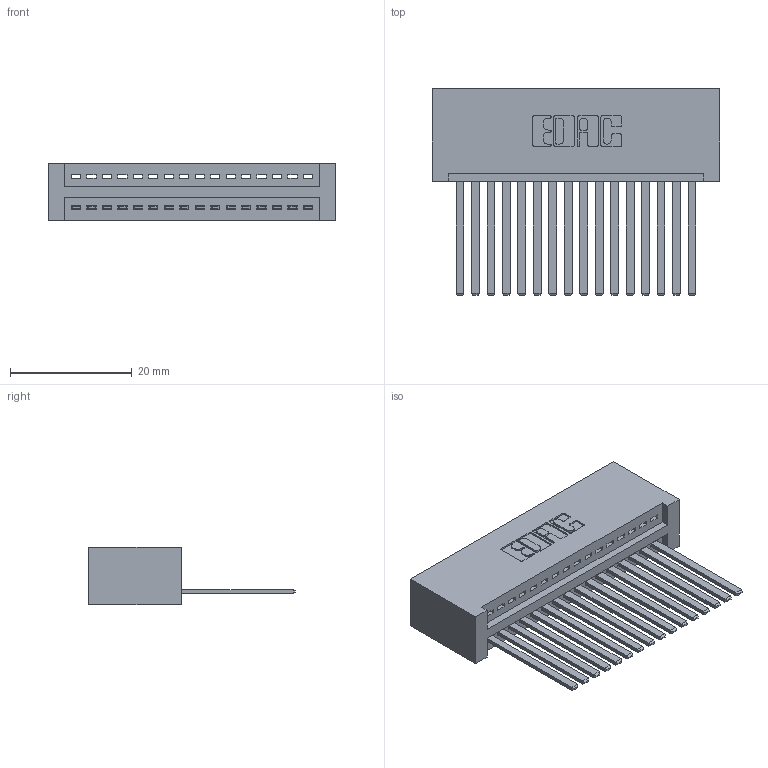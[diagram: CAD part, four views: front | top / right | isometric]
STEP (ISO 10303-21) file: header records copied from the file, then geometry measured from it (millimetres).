
FILE_DESCRIPTION (( 'STEP AP203' ), '1' );
FILE_NAME ('345-016-544-101.STEP', '2018-08-19T00:21:24', ( '' ), ( '' ), 'SwSTEP 2.0', 'SolidWorks 2016', '' );
FILE_SCHEMA (( 'CONFIG_CONTROL_DESIGN' ));
Length unit declared in the file: inch
Products named in the file (3): 345 Part_No Mounting Lugs; 345-292-001_345-293-144; 345-016-544-101
Assembly tree (17 placements, depth 2):
  345-016-544-101
    345 Part_No Mounting Lugs
    345-292-001_345-293-144  x16
Bounding box: 47.24 x 33.96 x 9.4 mm (x, y, z)
Volume: 5044 mm3; surface area: 7096 mm2
Topology: 17 solids, 17 shells, 950 faces, 2845 edges, 1874 vertices
Faces by surface type: plane 652, cylinder 298
Entity records: 15081 total; most frequent: CARTESIAN_POINT 2620, ORIENTED_EDGE 2570, DIRECTION 2317, EDGE_CURVE 1285, LINE 1101, VECTOR 1101, VERTEX_POINT 854, AXIS2_PLACEMENT_3D 608
